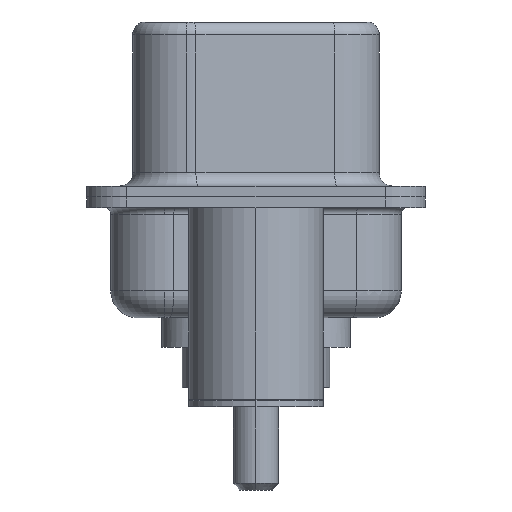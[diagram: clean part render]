
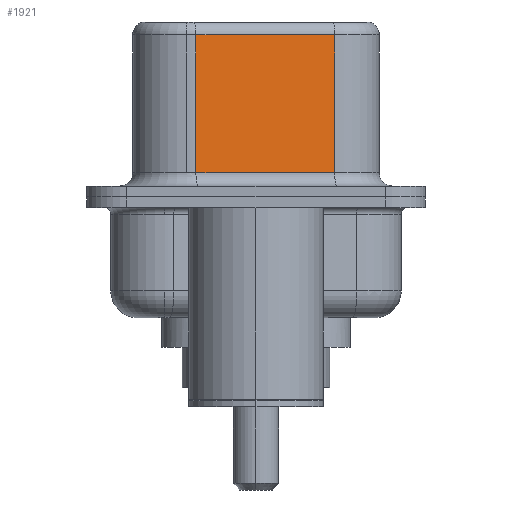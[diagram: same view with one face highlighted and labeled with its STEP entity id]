
A CAD part, left-side view. The second image highlights one B-rep face of the part: STEP entity #1921.
In plain terms, the highlighted planar face has unit normal (-0.985, -0.174, 0).
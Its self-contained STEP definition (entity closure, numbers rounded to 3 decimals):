
#27 = ORIENTED_EDGE ( 'NONE', *, *, #7296, .T. ) ;
#650 = LINE ( 'NONE', #6840, #14689 ) ;
#1303 = CARTESIAN_POINT ( 'NONE',  ( 4.565, -2.927, 6.52 ) ) ;
#1921 = ADVANCED_FACE ( 'NONE', ( #12209 ), #12611, .F. ) ;
#2092 = AXIS2_PLACEMENT_3D ( 'NONE', #15361, #3448, #16539 ) ;
#2615 = DIRECTION ( 'NONE',  ( 0., 0., -1. ) ) ;
#3434 = ORIENTED_EDGE ( 'NONE', *, *, #15891, .T. ) ;
#3448 = DIRECTION ( 'NONE',  ( 0.985, 0.174, 0. ) ) ;
#3485 = CARTESIAN_POINT ( 'NONE',  ( 4.565, -2.927, 6.02 ) ) ;
#3995 = CARTESIAN_POINT ( 'NONE',  ( 4.565, -2.927, 6.02 ) ) ;
#4181 = DIRECTION ( 'NONE',  ( 0.174, -0.985, 0. ) ) ;
#5295 = VERTEX_POINT ( 'NONE', #5556 ) ;
#5556 = CARTESIAN_POINT ( 'NONE',  ( 4.565, -2.927, 0.9 ) ) ;
#6125 = DIRECTION ( 'NONE',  ( -0.174, 0.985, 0. ) ) ;
#6166 = EDGE_CURVE ( 'NONE', #10786, #9821, #12936, .T. ) ;
#6280 = ORIENTED_EDGE ( 'NONE', *, *, #6166, .T. ) ;
#6552 = CARTESIAN_POINT ( 'NONE',  ( 3.655, 2.233, 6.52 ) ) ;
#6840 = CARTESIAN_POINT ( 'NONE',  ( 4.565, -2.927, 0.9 ) ) ;
#7249 = DIRECTION ( 'NONE',  ( 0., 0., -1. ) ) ;
#7296 = EDGE_CURVE ( 'NONE', #13749, #10786, #16400, .T. ) ;
#8472 = ORIENTED_EDGE ( 'NONE', *, *, #13249, .F. ) ;
#8677 = VECTOR ( 'NONE', #2615, 1000. ) ;
#9347 = VECTOR ( 'NONE', #7249, 1000. ) ;
#9821 = VERTEX_POINT ( 'NONE', #13259 ) ;
#10786 = VERTEX_POINT ( 'NONE', #11125 ) ;
#11125 = CARTESIAN_POINT ( 'NONE',  ( 3.655, 2.233, 6.02 ) ) ;
#12209 = FACE_OUTER_BOUND ( 'NONE', #17113, .T. ) ;
#12246 = LINE ( 'NONE', #1303, #8677 ) ;
#12611 = PLANE ( 'NONE',  #2092 ) ;
#12909 = VECTOR ( 'NONE', #6125, 1000. ) ;
#12936 = LINE ( 'NONE', #6552, #9347 ) ;
#13249 = EDGE_CURVE ( 'NONE', #13749, #5295, #12246, .T. ) ;
#13259 = CARTESIAN_POINT ( 'NONE',  ( 3.655, 2.233, 0.9 ) ) ;
#13749 = VERTEX_POINT ( 'NONE', #3995 ) ;
#14689 = VECTOR ( 'NONE', #4181, 1000. ) ;
#15361 = CARTESIAN_POINT ( 'NONE',  ( 4.565, -2.927, 6.52 ) ) ;
#15891 = EDGE_CURVE ( 'NONE', #9821, #5295, #650, .T. ) ;
#16400 = LINE ( 'NONE', #3485, #12909 ) ;
#16539 = DIRECTION ( 'NONE',  ( -0.174, 0.985, 0. ) ) ;
#17113 = EDGE_LOOP ( 'NONE', ( #8472, #27, #6280, #3434 ) ) ;
